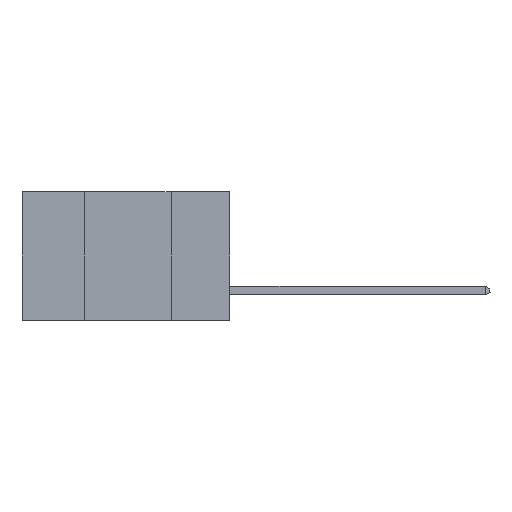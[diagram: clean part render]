
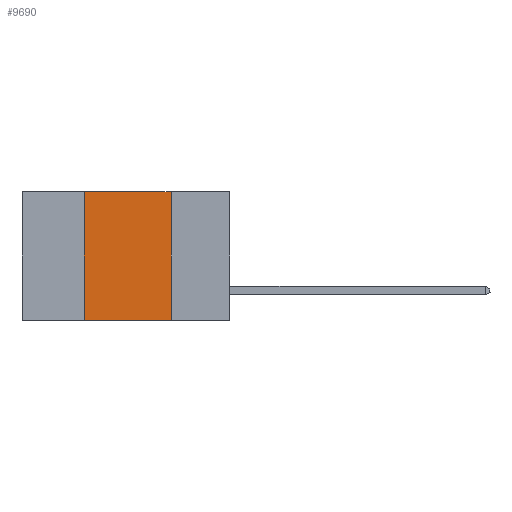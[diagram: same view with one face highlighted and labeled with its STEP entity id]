
A CAD part, left-side view. The second image highlights one B-rep face of the part: STEP entity #9690.
In plain terms, the highlighted planar face has unit normal (-1, 0, 0).
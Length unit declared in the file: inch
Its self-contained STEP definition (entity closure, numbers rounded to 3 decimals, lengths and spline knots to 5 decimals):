
#242 = DIRECTION ( 'NONE',  ( 0., -1., 0. ) ) ;
#980 = CARTESIAN_POINT ( 'NONE',  ( 0., 0.17, 0. ) ) ;
#1150 = DIRECTION ( 'NONE',  ( 0., 0., -1. ) ) ;
#1173 = CARTESIAN_POINT ( 'NONE',  ( 0., 0.17, -0.37 ) ) ;
#1667 = EDGE_CURVE ( 'NONE', #9235, #5801, #22510, .T. ) ;
#1739 = CARTESIAN_POINT ( 'NONE',  ( 0., 0.6, 0. ) ) ;
#1757 = CARTESIAN_POINT ( 'NONE',  ( 0., 0.42, 0. ) ) ;
#1886 = CARTESIAN_POINT ( 'NONE',  ( 0., 0.42, -0.37 ) ) ;
#2660 = ORIENTED_EDGE ( 'NONE', *, *, #1667, .F. ) ;
#4101 = VECTOR ( 'NONE', #23015, 39.37008 ) ;
#4406 = LINE ( 'NONE', #1757, #4101 ) ;
#4934 = DIRECTION ( 'NONE',  ( 1., 0., 0. ) ) ;
#5181 = CARTESIAN_POINT ( 'NONE',  ( 0., 0.6, 0. ) ) ;
#5479 = LINE ( 'NONE', #1739, #22665 ) ;
#5801 = VERTEX_POINT ( 'NONE', #1173 ) ;
#5915 = VECTOR ( 'NONE', #1150, 39.37008 ) ;
#7031 = PLANE ( 'NONE',  #14185 ) ;
#8062 = CARTESIAN_POINT ( 'NONE',  ( 0., 0.42, 0. ) ) ;
#9235 = VERTEX_POINT ( 'NONE', #12721 ) ;
#9284 = VERTEX_POINT ( 'NONE', #1886 ) ;
#9690 = ADVANCED_FACE ( 'NONE', ( #14770 ), #7031, .F. ) ;
#10653 = LINE ( 'NONE', #24384, #17844 ) ;
#12721 = CARTESIAN_POINT ( 'NONE',  ( 0., 0.17, 0. ) ) ;
#12908 = EDGE_CURVE ( 'NONE', #9284, #21784, #4406, .T. ) ;
#14185 = AXIS2_PLACEMENT_3D ( 'NONE', #5181, #4934, #22455 ) ;
#14428 = ORIENTED_EDGE ( 'NONE', *, *, #22153, .F. ) ;
#14770 = FACE_OUTER_BOUND ( 'NONE', #22625, .T. ) ;
#15047 = EDGE_CURVE ( 'NONE', #9284, #5801, #10653, .T. ) ;
#17844 = VECTOR ( 'NONE', #19162, 39.37008 ) ;
#17918 = ORIENTED_EDGE ( 'NONE', *, *, #15047, .T. ) ;
#19162 = DIRECTION ( 'NONE',  ( 0., -1., 0. ) ) ;
#21784 = VERTEX_POINT ( 'NONE', #8062 ) ;
#22153 = EDGE_CURVE ( 'NONE', #21784, #9235, #5479, .T. ) ;
#22455 = DIRECTION ( 'NONE',  ( 0., 0., -1. ) ) ;
#22510 = LINE ( 'NONE', #980, #5915 ) ;
#22625 = EDGE_LOOP ( 'NONE', ( #2660, #14428, #23617, #17918 ) ) ;
#22665 = VECTOR ( 'NONE', #242, 39.37008 ) ;
#23015 = DIRECTION ( 'NONE',  ( 0., 0., 1. ) ) ;
#23617 = ORIENTED_EDGE ( 'NONE', *, *, #12908, .F. ) ;
#24384 = CARTESIAN_POINT ( 'NONE',  ( 0., 0.6, -0.37 ) ) ;
